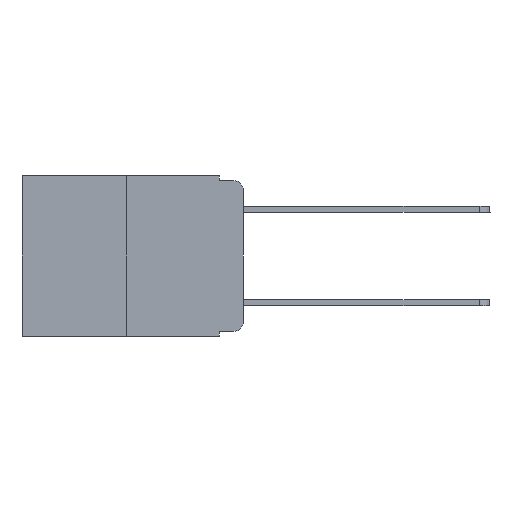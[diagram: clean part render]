
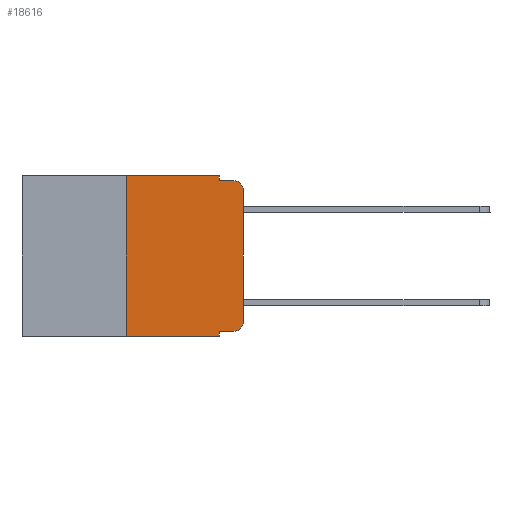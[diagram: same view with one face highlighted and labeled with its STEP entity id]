
A CAD part, left-side view. The second image highlights one B-rep face of the part: STEP entity #18616.
In plain terms, the highlighted planar face has unit normal (-1, 0, 0).
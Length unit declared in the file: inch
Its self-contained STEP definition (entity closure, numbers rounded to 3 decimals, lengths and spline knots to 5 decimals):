
#253 = VERTEX_POINT ( 'NONE', #13854 ) ;
#297 = CARTESIAN_POINT ( 'NONE',  ( 0., 0.051, -0.343 ) ) ;
#318 = CARTESIAN_POINT ( 'NONE',  ( 0., 0., 0. ) ) ;
#401 = VERTEX_POINT ( 'NONE', #6904 ) ;
#1082 = ORIENTED_EDGE ( 'NONE', *, *, #6480, .T. ) ;
#1130 = DIRECTION ( 'NONE',  ( 0., -1., 0. ) ) ;
#1364 = CARTESIAN_POINT ( 'NONE',  ( 0., 0., -0.313 ) ) ;
#1475 = EDGE_LOOP ( 'NONE', ( #13265, #10804, #12513, #2656, #4099, #13951, #5282, #6042, #1082, #12345 ) ) ;
#1559 = LINE ( 'NONE', #14724, #16680 ) ;
#1614 = EDGE_CURVE ( 'NONE', #18545, #10322, #6957, .T. ) ;
#1669 = CARTESIAN_POINT ( 'NONE',  ( 0., 0.02, -0.03 ) ) ;
#1826 = AXIS2_PLACEMENT_3D ( 'NONE', #18059, #15215, #16683 ) ;
#1847 = DIRECTION ( 'NONE',  ( 0., 0., -1. ) ) ;
#1861 = EDGE_CURVE ( 'NONE', #9250, #17311, #11540, .T. ) ;
#2508 = LINE ( 'NONE', #8060, #9690 ) ;
#2656 = ORIENTED_EDGE ( 'NONE', *, *, #4100, .F. ) ;
#2939 = CARTESIAN_POINT ( 'NONE',  ( 0., 0.02, -0.01 ) ) ;
#3380 = DIRECTION ( 'NONE',  ( 0., 0., -1. ) ) ;
#3711 = VECTOR ( 'NONE', #18700, 39.37008 ) ;
#3746 = DIRECTION ( 'NONE',  ( 0., 0., -1. ) ) ;
#3833 = EDGE_CURVE ( 'NONE', #16838, #10322, #16546, .T. ) ;
#3932 = CARTESIAN_POINT ( 'NONE',  ( 0., 0.473, -0.343 ) ) ;
#4079 = VECTOR ( 'NONE', #7644, 39.37008 ) ;
#4099 = ORIENTED_EDGE ( 'NONE', *, *, #4132, .F. ) ;
#4100 = EDGE_CURVE ( 'NONE', #15212, #16838, #15390, .T. ) ;
#4132 = EDGE_CURVE ( 'NONE', #14797, #15212, #16980, .T. ) ;
#4176 = CARTESIAN_POINT ( 'NONE',  ( 0., 0.25, -0.343 ) ) ;
#5132 = DIRECTION ( 'NONE',  ( 1., 0., 0. ) ) ;
#5220 = CARTESIAN_POINT ( 'NONE',  ( 0., 0.051, 0. ) ) ;
#5282 = ORIENTED_EDGE ( 'NONE', *, *, #1861, .T. ) ;
#5771 = CARTESIAN_POINT ( 'NONE',  ( 0., 0.051, -0.01 ) ) ;
#5909 = DIRECTION ( 'NONE',  ( 0., -1., 0. ) ) ;
#6042 = ORIENTED_EDGE ( 'NONE', *, *, #9583, .F. ) ;
#6480 = EDGE_CURVE ( 'NONE', #401, #253, #1559, .T. ) ;
#6904 = CARTESIAN_POINT ( 'NONE',  ( 0., 0.051, -0.333 ) ) ;
#6957 = CIRCLE ( 'NONE', #9030, 0.02 ) ;
#7644 = DIRECTION ( 'NONE',  ( 0., 0., 1. ) ) ;
#8009 = AXIS2_PLACEMENT_3D ( 'NONE', #16676, #5132, #11159 ) ;
#8060 = CARTESIAN_POINT ( 'NONE',  ( 0., 0.051, 0. ) ) ;
#8331 = LINE ( 'NONE', #9987, #15281 ) ;
#9030 = AXIS2_PLACEMENT_3D ( 'NONE', #1669, #16396, #1847 ) ;
#9250 = VERTEX_POINT ( 'NONE', #4176 ) ;
#9342 = PLANE ( 'NONE',  #8009 ) ;
#9583 = EDGE_CURVE ( 'NONE', #401, #17311, #2508, .T. ) ;
#9690 = VECTOR ( 'NONE', #3746, 39.37008 ) ;
#9987 = CARTESIAN_POINT ( 'NONE',  ( 0., 0.25, 0. ) ) ;
#10322 = VERTEX_POINT ( 'NONE', #2939 ) ;
#10569 = DIRECTION ( 'NONE',  ( 0., -1., 0. ) ) ;
#10706 = CARTESIAN_POINT ( 'NONE',  ( 0., 0., -0.03 ) ) ;
#10804 = ORIENTED_EDGE ( 'NONE', *, *, #1614, .T. ) ;
#10997 = EDGE_CURVE ( 'NONE', #253, #11282, #12979, .T. ) ;
#11159 = DIRECTION ( 'NONE',  ( 0., 0., -1. ) ) ;
#11282 = VERTEX_POINT ( 'NONE', #1364 ) ;
#11540 = LINE ( 'NONE', #3932, #14999 ) ;
#12034 = CARTESIAN_POINT ( 'NONE',  ( 0., 0.051, 0. ) ) ;
#12345 = ORIENTED_EDGE ( 'NONE', *, *, #10997, .T. ) ;
#12513 = ORIENTED_EDGE ( 'NONE', *, *, #3833, .F. ) ;
#12979 = CIRCLE ( 'NONE', #1826, 0.02 ) ;
#13265 = ORIENTED_EDGE ( 'NONE', *, *, #16754, .T. ) ;
#13306 = VECTOR ( 'NONE', #10569, 39.37008 ) ;
#13854 = CARTESIAN_POINT ( 'NONE',  ( 0., 0.02, -0.333 ) ) ;
#13951 = ORIENTED_EDGE ( 'NONE', *, *, #17995, .F. ) ;
#14204 = CARTESIAN_POINT ( 'NONE',  ( 0., 0.25, 0. ) ) ;
#14559 = DIRECTION ( 'NONE',  ( 0., 0., 1. ) ) ;
#14724 = CARTESIAN_POINT ( 'NONE',  ( 0., 0.051, -0.333 ) ) ;
#14797 = VERTEX_POINT ( 'NONE', #14204 ) ;
#14999 = VECTOR ( 'NONE', #1130, 39.37008 ) ;
#15212 = VERTEX_POINT ( 'NONE', #5220 ) ;
#15215 = DIRECTION ( 'NONE',  ( -1., 0., 0. ) ) ;
#15281 = VECTOR ( 'NONE', #14559, 39.37008 ) ;
#15390 = LINE ( 'NONE', #12034, #17661 ) ;
#15437 = CARTESIAN_POINT ( 'NONE',  ( 0., 0.051, -0.01 ) ) ;
#16396 = DIRECTION ( 'NONE',  ( -1., 0., 0. ) ) ;
#16546 = LINE ( 'NONE', #5771, #3711 ) ;
#16676 = CARTESIAN_POINT ( 'NONE',  ( 0., 0.473, 0. ) ) ;
#16680 = VECTOR ( 'NONE', #5909, 39.37008 ) ;
#16683 = DIRECTION ( 'NONE',  ( 0., 0., -1. ) ) ;
#16684 = LINE ( 'NONE', #318, #4079 ) ;
#16754 = EDGE_CURVE ( 'NONE', #11282, #18545, #16684, .T. ) ;
#16838 = VERTEX_POINT ( 'NONE', #15437 ) ;
#16980 = LINE ( 'NONE', #17985, #13306 ) ;
#17311 = VERTEX_POINT ( 'NONE', #297 ) ;
#17661 = VECTOR ( 'NONE', #3380, 39.37008 ) ;
#17985 = CARTESIAN_POINT ( 'NONE',  ( 0., 0.473, 0. ) ) ;
#17995 = EDGE_CURVE ( 'NONE', #9250, #14797, #8331, .T. ) ;
#18059 = CARTESIAN_POINT ( 'NONE',  ( 0., 0.02, -0.313 ) ) ;
#18217 = FACE_OUTER_BOUND ( 'NONE', #1475, .T. ) ;
#18545 = VERTEX_POINT ( 'NONE', #10706 ) ;
#18616 = ADVANCED_FACE ( 'NONE', ( #18217 ), #9342, .F. ) ;
#18700 = DIRECTION ( 'NONE',  ( 0., -1., 0. ) ) ;
